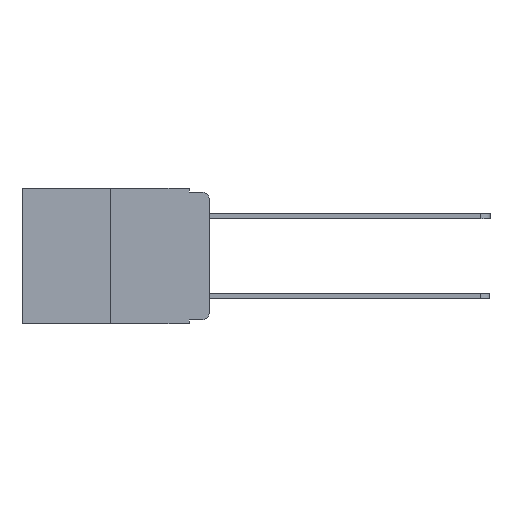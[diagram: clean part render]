
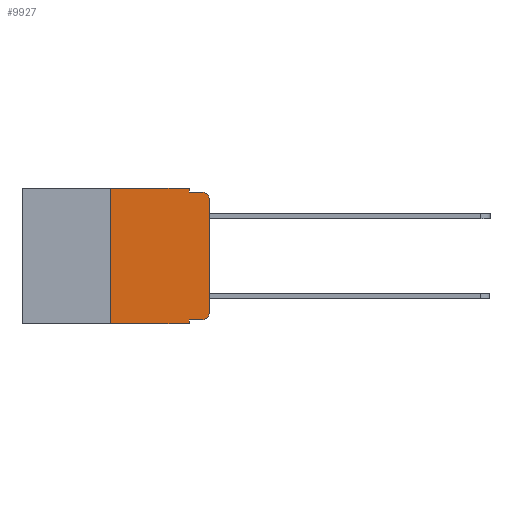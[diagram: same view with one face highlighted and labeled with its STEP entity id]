
A CAD part, left-side view. The second image highlights one B-rep face of the part: STEP entity #9927.
In plain terms, the highlighted planar face has unit normal (-1, 0, 0).
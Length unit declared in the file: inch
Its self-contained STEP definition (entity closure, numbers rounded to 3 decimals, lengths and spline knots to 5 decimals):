
#230 = DIRECTION ( 'NONE',  ( 0., 0., -1. ) ) ;
#335 = VERTEX_POINT ( 'NONE', #3120 ) ;
#396 = CARTESIAN_POINT ( 'NONE',  ( 0., 0.051, 0. ) ) ;
#1045 = LINE ( 'NONE', #11287, #9185 ) ;
#1552 = VECTOR ( 'NONE', #4121, 39.37008 ) ;
#1924 = CARTESIAN_POINT ( 'NONE',  ( 0., 0., -0.03 ) ) ;
#2020 = VERTEX_POINT ( 'NONE', #396 ) ;
#2083 = VERTEX_POINT ( 'NONE', #1924 ) ;
#2390 = PLANE ( 'NONE',  #12526 ) ;
#3120 = CARTESIAN_POINT ( 'NONE',  ( 0., 0.02, -0.01 ) ) ;
#3161 = EDGE_CURVE ( 'NONE', #16330, #2083, #17547, .T. ) ;
#3214 = LINE ( 'NONE', #11583, #18445 ) ;
#3417 = EDGE_CURVE ( 'NONE', #3824, #4869, #13924, .T. ) ;
#3758 = CARTESIAN_POINT ( 'NONE',  ( 0., 0., 0. ) ) ;
#3824 = VERTEX_POINT ( 'NONE', #18897 ) ;
#4121 = DIRECTION ( 'NONE',  ( 0., 0., 1. ) ) ;
#4147 = ORIENTED_EDGE ( 'NONE', *, *, #3417, .T. ) ;
#4355 = EDGE_CURVE ( 'NONE', #16948, #16330, #9093, .T. ) ;
#4391 = ORIENTED_EDGE ( 'NONE', *, *, #15453, .F. ) ;
#4700 = VECTOR ( 'NONE', #19570, 39.37008 ) ;
#4869 = VERTEX_POINT ( 'NONE', #13744 ) ;
#4912 = CARTESIAN_POINT ( 'NONE',  ( 0., 0.02, -0.313 ) ) ;
#5304 = DIRECTION ( 'NONE',  ( -1., 0., 0. ) ) ;
#5603 = CARTESIAN_POINT ( 'NONE',  ( 0., 0.051, 0. ) ) ;
#5627 = DIRECTION ( 'NONE',  ( 1., 0., 0. ) ) ;
#6098 = ORIENTED_EDGE ( 'NONE', *, *, #16928, .F. ) ;
#6225 = ORIENTED_EDGE ( 'NONE', *, *, #17404, .F. ) ;
#6484 = DIRECTION ( 'NONE',  ( 0., 0., -1. ) ) ;
#6612 = ORIENTED_EDGE ( 'NONE', *, *, #6985, .F. ) ;
#6860 = EDGE_LOOP ( 'NONE', ( #19227, #9309, #6098, #13661, #6612, #4391, #4147, #6225, #8643, #9654 ) ) ;
#6985 = EDGE_CURVE ( 'NONE', #12631, #2020, #9638, .T. ) ;
#7165 = DIRECTION ( 'NONE',  ( 0., 0., -1. ) ) ;
#7738 = CARTESIAN_POINT ( 'NONE',  ( 0., 0.02, -0.333 ) ) ;
#7871 = LINE ( 'NONE', #5603, #15497 ) ;
#8643 = ORIENTED_EDGE ( 'NONE', *, *, #18913, .T. ) ;
#9039 = FACE_OUTER_BOUND ( 'NONE', #6860, .T. ) ;
#9093 = CIRCLE ( 'NONE', #12458, 0.02 ) ;
#9185 = VECTOR ( 'NONE', #12846, 39.37008 ) ;
#9309 = ORIENTED_EDGE ( 'NONE', *, *, #15938, .T. ) ;
#9638 = LINE ( 'NONE', #10952, #17108 ) ;
#9654 = ORIENTED_EDGE ( 'NONE', *, *, #4355, .T. ) ;
#9927 = ADVANCED_FACE ( 'NONE', ( #9039 ), #2390, .F. ) ;
#10952 = CARTESIAN_POINT ( 'NONE',  ( 0., 0.473, 0. ) ) ;
#11287 = CARTESIAN_POINT ( 'NONE',  ( 0., 0.25, 0. ) ) ;
#11583 = CARTESIAN_POINT ( 'NONE',  ( 0., 0.051, 0. ) ) ;
#12121 = CARTESIAN_POINT ( 'NONE',  ( 0., 0.051, -0.333 ) ) ;
#12214 = VECTOR ( 'NONE', #19326, 39.37008 ) ;
#12280 = CARTESIAN_POINT ( 'NONE',  ( 0., 0.473, -0.343 ) ) ;
#12305 = CIRCLE ( 'NONE', #18635, 0.02 ) ;
#12423 = CARTESIAN_POINT ( 'NONE',  ( 0., 0.25, 0. ) ) ;
#12458 = AXIS2_PLACEMENT_3D ( 'NONE', #4912, #15648, #6484 ) ;
#12506 = DIRECTION ( 'NONE',  ( 0., -1., 0. ) ) ;
#12526 = AXIS2_PLACEMENT_3D ( 'NONE', #14857, #5627, #16319 ) ;
#12631 = VERTEX_POINT ( 'NONE', #12423 ) ;
#12846 = DIRECTION ( 'NONE',  ( 0., 0., 1. ) ) ;
#13029 = EDGE_CURVE ( 'NONE', #2020, #16168, #3214, .T. ) ;
#13530 = CARTESIAN_POINT ( 'NONE',  ( 0., 0.051, -0.01 ) ) ;
#13661 = ORIENTED_EDGE ( 'NONE', *, *, #13029, .F. ) ;
#13744 = CARTESIAN_POINT ( 'NONE',  ( 0., 0.051, -0.343 ) ) ;
#13848 = CARTESIAN_POINT ( 'NONE',  ( 0., 0., -0.313 ) ) ;
#13924 = LINE ( 'NONE', #12280, #17329 ) ;
#14314 = VERTEX_POINT ( 'NONE', #17712 ) ;
#14551 = CARTESIAN_POINT ( 'NONE',  ( 0., 0.02, -0.03 ) ) ;
#14857 = CARTESIAN_POINT ( 'NONE',  ( 0., 0.473, 0. ) ) ;
#15238 = DIRECTION ( 'NONE',  ( 0., -1., 0. ) ) ;
#15453 = EDGE_CURVE ( 'NONE', #3824, #12631, #1045, .T. ) ;
#15497 = VECTOR ( 'NONE', #7165, 39.37008 ) ;
#15648 = DIRECTION ( 'NONE',  ( -1., 0., 0. ) ) ;
#15938 = EDGE_CURVE ( 'NONE', #2083, #335, #12305, .T. ) ;
#15996 = DIRECTION ( 'NONE',  ( 0., 0., -1. ) ) ;
#16126 = LINE ( 'NONE', #12121, #12214 ) ;
#16168 = VERTEX_POINT ( 'NONE', #13530 ) ;
#16319 = DIRECTION ( 'NONE',  ( 0., 0., -1. ) ) ;
#16330 = VERTEX_POINT ( 'NONE', #13848 ) ;
#16439 = LINE ( 'NONE', #18162, #4700 ) ;
#16928 = EDGE_CURVE ( 'NONE', #16168, #335, #16439, .T. ) ;
#16948 = VERTEX_POINT ( 'NONE', #7738 ) ;
#17108 = VECTOR ( 'NONE', #12506, 39.37008 ) ;
#17329 = VECTOR ( 'NONE', #15238, 39.37008 ) ;
#17404 = EDGE_CURVE ( 'NONE', #14314, #4869, #7871, .T. ) ;
#17547 = LINE ( 'NONE', #3758, #1552 ) ;
#17712 = CARTESIAN_POINT ( 'NONE',  ( 0., 0.051, -0.333 ) ) ;
#18162 = CARTESIAN_POINT ( 'NONE',  ( 0., 0.051, -0.01 ) ) ;
#18445 = VECTOR ( 'NONE', #230, 39.37008 ) ;
#18635 = AXIS2_PLACEMENT_3D ( 'NONE', #14551, #5304, #15996 ) ;
#18897 = CARTESIAN_POINT ( 'NONE',  ( 0., 0.25, -0.343 ) ) ;
#18913 = EDGE_CURVE ( 'NONE', #14314, #16948, #16126, .T. ) ;
#19227 = ORIENTED_EDGE ( 'NONE', *, *, #3161, .T. ) ;
#19326 = DIRECTION ( 'NONE',  ( 0., -1., 0. ) ) ;
#19570 = DIRECTION ( 'NONE',  ( 0., -1., 0. ) ) ;
